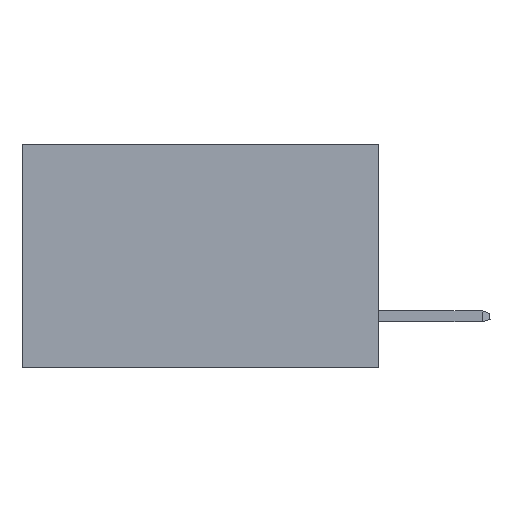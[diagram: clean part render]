
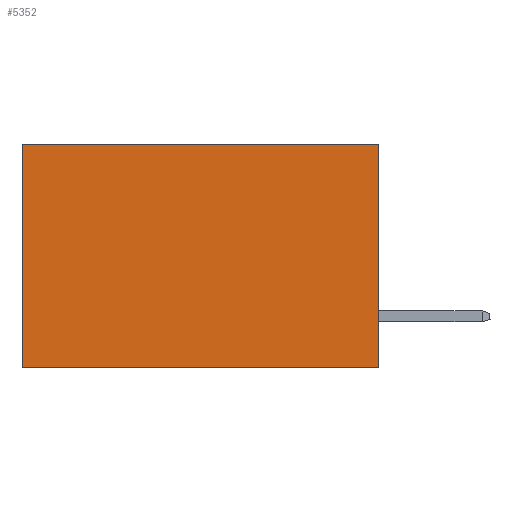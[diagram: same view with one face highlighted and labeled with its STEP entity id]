
A CAD part, left-side view. The second image highlights one B-rep face of the part: STEP entity #5352.
In plain terms, the highlighted planar face has unit normal (-1, 0, 0).
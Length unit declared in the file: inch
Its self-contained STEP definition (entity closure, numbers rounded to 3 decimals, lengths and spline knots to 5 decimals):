
#42 = LINE ( 'NONE', #7223, #9187 ) ;
#496 = DIRECTION ( 'NONE',  ( 0., 1., 0. ) ) ;
#3511 = CARTESIAN_POINT ( 'NONE',  ( 0.277, 0., -0.37 ) ) ;
#4915 = ORIENTED_EDGE ( 'NONE', *, *, #21975, .F. ) ;
#5352 = ADVANCED_FACE ( 'NONE', ( #24752 ), #10101, .F. ) ;
#5730 = VERTEX_POINT ( 'NONE', #3511 ) ;
#6382 = AXIS2_PLACEMENT_3D ( 'NONE', #18539, #9696, #9631 ) ;
#7223 = CARTESIAN_POINT ( 'NONE',  ( 0.277, 0., -0.37 ) ) ;
#7290 = CARTESIAN_POINT ( 'NONE',  ( 0.277, 0.59, 0. ) ) ;
#7646 = LINE ( 'NONE', #25875, #17973 ) ;
#9187 = VECTOR ( 'NONE', #27415, 39.37008 ) ;
#9631 = DIRECTION ( 'NONE',  ( 0., 0., -1. ) ) ;
#9696 = DIRECTION ( 'NONE',  ( 1., 0., 0. ) ) ;
#10101 = PLANE ( 'NONE',  #6382 ) ;
#10304 = VECTOR ( 'NONE', #15957, 39.37008 ) ;
#11188 = LINE ( 'NONE', #26468, #23895 ) ;
#12754 = EDGE_CURVE ( 'NONE', #21659, #27959, #7646, .T. ) ;
#13410 = CARTESIAN_POINT ( 'NONE',  ( 0.277, 0.59, -0.37 ) ) ;
#14452 = EDGE_LOOP ( 'NONE', ( #17950, #4915, #29264, #22547 ) ) ;
#15525 = EDGE_CURVE ( 'NONE', #21659, #5730, #11188, .T. ) ;
#15957 = DIRECTION ( 'NONE',  ( 0., 0., -1. ) ) ;
#16818 = CARTESIAN_POINT ( 'NONE',  ( 0.277, 0.59, -0.37 ) ) ;
#17950 = ORIENTED_EDGE ( 'NONE', *, *, #22891, .T. ) ;
#17973 = VECTOR ( 'NONE', #496, 39.37008 ) ;
#18539 = CARTESIAN_POINT ( 'NONE',  ( 0.277, 0., -0.37 ) ) ;
#18556 = CARTESIAN_POINT ( 'NONE',  ( 0.277, 0., 0. ) ) ;
#21659 = VERTEX_POINT ( 'NONE', #18556 ) ;
#21975 = EDGE_CURVE ( 'NONE', #5730, #29036, #42, .T. ) ;
#22547 = ORIENTED_EDGE ( 'NONE', *, *, #12754, .T. ) ;
#22891 = EDGE_CURVE ( 'NONE', #27959, #29036, #30328, .T. ) ;
#23895 = VECTOR ( 'NONE', #28927, 39.37008 ) ;
#24752 = FACE_OUTER_BOUND ( 'NONE', #14452, .T. ) ;
#25875 = CARTESIAN_POINT ( 'NONE',  ( 0.277, 0., 0. ) ) ;
#26468 = CARTESIAN_POINT ( 'NONE',  ( 0.277, 0., -0.37 ) ) ;
#27415 = DIRECTION ( 'NONE',  ( 0., 1., 0. ) ) ;
#27959 = VERTEX_POINT ( 'NONE', #7290 ) ;
#28927 = DIRECTION ( 'NONE',  ( 0., 0., -1. ) ) ;
#29036 = VERTEX_POINT ( 'NONE', #16818 ) ;
#29264 = ORIENTED_EDGE ( 'NONE', *, *, #15525, .F. ) ;
#30328 = LINE ( 'NONE', #13410, #10304 ) ;
